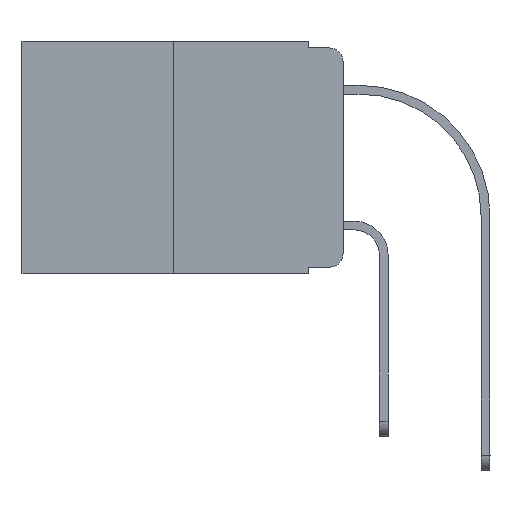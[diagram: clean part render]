
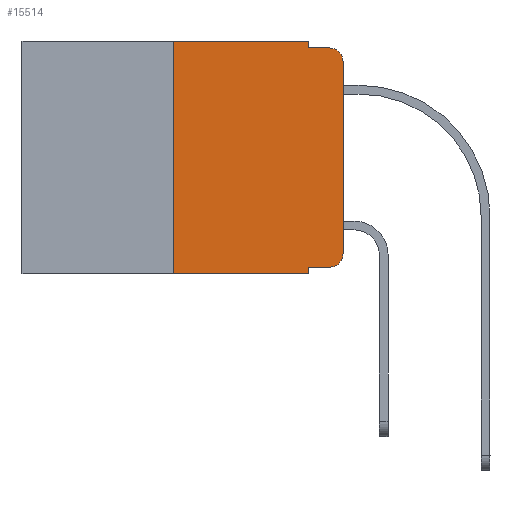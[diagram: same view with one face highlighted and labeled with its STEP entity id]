
A CAD part, left-side view. The second image highlights one B-rep face of the part: STEP entity #15514.
In plain terms, the highlighted planar face has unit normal (-1, 0, 0).
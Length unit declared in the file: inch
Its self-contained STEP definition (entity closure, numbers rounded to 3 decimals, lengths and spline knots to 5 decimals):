
#67 = CARTESIAN_POINT ( 'NONE',  ( 0., 0.25, 0. ) ) ;
#477 = VERTEX_POINT ( 'NONE', #18284 ) ;
#546 = VERTEX_POINT ( 'NONE', #12119 ) ;
#637 = AXIS2_PLACEMENT_3D ( 'NONE', #7816, #9800, #1128 ) ;
#1009 = EDGE_CURVE ( 'NONE', #4754, #14973, #13882, .T. ) ;
#1128 = DIRECTION ( 'NONE',  ( 0., 0., -1. ) ) ;
#1262 = ORIENTED_EDGE ( 'NONE', *, *, #1712, .F. ) ;
#1712 = EDGE_CURVE ( 'NONE', #546, #15077, #9567, .T. ) ;
#1835 = EDGE_CURVE ( 'NONE', #15077, #17158, #16904, .T. ) ;
#2185 = ORIENTED_EDGE ( 'NONE', *, *, #1835, .F. ) ;
#2473 = CARTESIAN_POINT ( 'NONE',  ( 0., 0.25, 0. ) ) ;
#2517 = AXIS2_PLACEMENT_3D ( 'NONE', #15129, #21877, #21555 ) ;
#3217 = ORIENTED_EDGE ( 'NONE', *, *, #8223, .T. ) ;
#3454 = CARTESIAN_POINT ( 'NONE',  ( 0., 0., -0.313 ) ) ;
#3474 = CIRCLE ( 'NONE', #637, 0.02 ) ;
#3776 = CARTESIAN_POINT ( 'NONE',  ( 0., 0.051, 0. ) ) ;
#4103 = CIRCLE ( 'NONE', #20048, 0.02 ) ;
#4134 = VERTEX_POINT ( 'NONE', #8737 ) ;
#4154 = VECTOR ( 'NONE', #19986, 39.37008 ) ;
#4468 = LINE ( 'NONE', #14695, #6755 ) ;
#4754 = VERTEX_POINT ( 'NONE', #19375 ) ;
#4858 = ORIENTED_EDGE ( 'NONE', *, *, #5311, .T. ) ;
#5140 = CARTESIAN_POINT ( 'NONE',  ( 0., 0.051, -0.01 ) ) ;
#5246 = CARTESIAN_POINT ( 'NONE',  ( 0., 0.02, -0.313 ) ) ;
#5311 = EDGE_CURVE ( 'NONE', #4134, #14973, #14889, .T. ) ;
#5994 = CARTESIAN_POINT ( 'NONE',  ( 0., 0., -0.03 ) ) ;
#6340 = ORIENTED_EDGE ( 'NONE', *, *, #14480, .T. ) ;
#6370 = ORIENTED_EDGE ( 'NONE', *, *, #21003, .T. ) ;
#6755 = VECTOR ( 'NONE', #18574, 39.37008 ) ;
#7177 = VERTEX_POINT ( 'NONE', #5994 ) ;
#7816 = CARTESIAN_POINT ( 'NONE',  ( 0., 0.02, -0.03 ) ) ;
#7995 = CARTESIAN_POINT ( 'NONE',  ( 0., 0.02, -0.01 ) ) ;
#8102 = CARTESIAN_POINT ( 'NONE',  ( 0., 0.473, -0.343 ) ) ;
#8223 = EDGE_CURVE ( 'NONE', #7177, #17158, #3474, .T. ) ;
#8737 = CARTESIAN_POINT ( 'NONE',  ( 0., 0.25, -0.343 ) ) ;
#9567 = LINE ( 'NONE', #13121, #16370 ) ;
#9582 = DIRECTION ( 'NONE',  ( 0., 0., 1. ) ) ;
#9800 = DIRECTION ( 'NONE',  ( -1., 0., 0. ) ) ;
#9987 = FACE_OUTER_BOUND ( 'NONE', #17499, .T. ) ;
#10764 = EDGE_CURVE ( 'NONE', #17306, #546, #4468, .T. ) ;
#11346 = LINE ( 'NONE', #16058, #18214 ) ;
#12119 = CARTESIAN_POINT ( 'NONE',  ( 0., 0.051, 0. ) ) ;
#12430 = DIRECTION ( 'NONE',  ( 0., 0., -1. ) ) ;
#12924 = LINE ( 'NONE', #2473, #21396 ) ;
#13054 = LINE ( 'NONE', #14624, #19602 ) ;
#13121 = CARTESIAN_POINT ( 'NONE',  ( 0., 0.051, 0. ) ) ;
#13182 = VECTOR ( 'NONE', #18572, 39.37008 ) ;
#13782 = CARTESIAN_POINT ( 'NONE',  ( 0., 0.051, -0.01 ) ) ;
#13882 = LINE ( 'NONE', #3776, #18124 ) ;
#14480 = EDGE_CURVE ( 'NONE', #4754, #477, #13054, .T. ) ;
#14494 = DIRECTION ( 'NONE',  ( 0., 0., 1. ) ) ;
#14624 = CARTESIAN_POINT ( 'NONE',  ( 0., 0.051, -0.333 ) ) ;
#14695 = CARTESIAN_POINT ( 'NONE',  ( 0., 0.473, 0. ) ) ;
#14797 = PLANE ( 'NONE',  #2517 ) ;
#14877 = EDGE_CURVE ( 'NONE', #4134, #17306, #12924, .T. ) ;
#14889 = LINE ( 'NONE', #8102, #4154 ) ;
#14909 = EDGE_CURVE ( 'NONE', #19722, #7177, #11346, .T. ) ;
#14973 = VERTEX_POINT ( 'NONE', #21792 ) ;
#15022 = ORIENTED_EDGE ( 'NONE', *, *, #14909, .T. ) ;
#15077 = VERTEX_POINT ( 'NONE', #5140 ) ;
#15129 = CARTESIAN_POINT ( 'NONE',  ( 0., 0.473, 0. ) ) ;
#15514 = ADVANCED_FACE ( 'NONE', ( #9987 ), #14797, .F. ) ;
#16058 = CARTESIAN_POINT ( 'NONE',  ( 0., 0., 0. ) ) ;
#16355 = DIRECTION ( 'NONE',  ( 0., 0., -1. ) ) ;
#16370 = VECTOR ( 'NONE', #16355, 39.37008 ) ;
#16904 = LINE ( 'NONE', #13782, #13182 ) ;
#17055 = ORIENTED_EDGE ( 'NONE', *, *, #10764, .F. ) ;
#17141 = DIRECTION ( 'NONE',  ( -1., 0., 0. ) ) ;
#17158 = VERTEX_POINT ( 'NONE', #7995 ) ;
#17306 = VERTEX_POINT ( 'NONE', #67 ) ;
#17499 = EDGE_LOOP ( 'NONE', ( #15022, #3217, #2185, #1262, #17055, #20049, #4858, #19794, #6340, #6370 ) ) ;
#18124 = VECTOR ( 'NONE', #12430, 39.37008 ) ;
#18214 = VECTOR ( 'NONE', #9582, 39.37008 ) ;
#18284 = CARTESIAN_POINT ( 'NONE',  ( 0., 0.02, -0.333 ) ) ;
#18572 = DIRECTION ( 'NONE',  ( 0., -1., 0. ) ) ;
#18574 = DIRECTION ( 'NONE',  ( 0., -1., 0. ) ) ;
#18916 = DIRECTION ( 'NONE',  ( 0., 0., -1. ) ) ;
#19375 = CARTESIAN_POINT ( 'NONE',  ( 0., 0.051, -0.333 ) ) ;
#19602 = VECTOR ( 'NONE', #21392, 39.37008 ) ;
#19722 = VERTEX_POINT ( 'NONE', #3454 ) ;
#19794 = ORIENTED_EDGE ( 'NONE', *, *, #1009, .F. ) ;
#19986 = DIRECTION ( 'NONE',  ( 0., -1., 0. ) ) ;
#20048 = AXIS2_PLACEMENT_3D ( 'NONE', #5246, #17141, #18916 ) ;
#20049 = ORIENTED_EDGE ( 'NONE', *, *, #14877, .F. ) ;
#21003 = EDGE_CURVE ( 'NONE', #477, #19722, #4103, .T. ) ;
#21392 = DIRECTION ( 'NONE',  ( 0., -1., 0. ) ) ;
#21396 = VECTOR ( 'NONE', #14494, 39.37008 ) ;
#21555 = DIRECTION ( 'NONE',  ( 0., 0., -1. ) ) ;
#21792 = CARTESIAN_POINT ( 'NONE',  ( 0., 0.051, -0.343 ) ) ;
#21877 = DIRECTION ( 'NONE',  ( 1., 0., 0. ) ) ;
